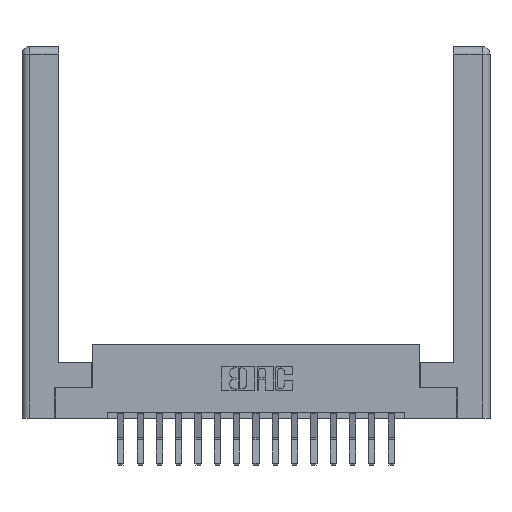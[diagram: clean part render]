
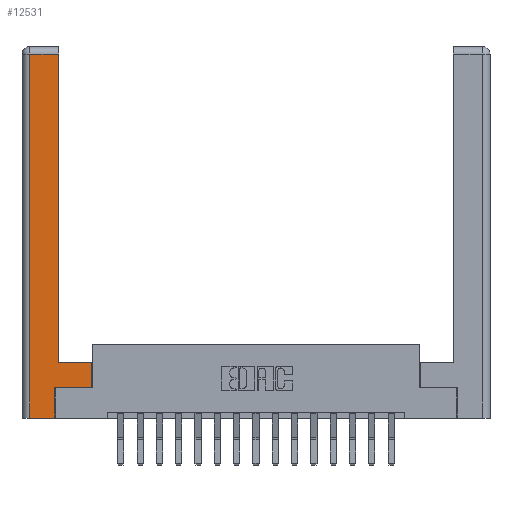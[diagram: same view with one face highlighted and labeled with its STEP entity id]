
A CAD part, top view. The second image highlights one B-rep face of the part: STEP entity #12531.
In plain terms, the highlighted planar face has unit normal (0, 0, 1).
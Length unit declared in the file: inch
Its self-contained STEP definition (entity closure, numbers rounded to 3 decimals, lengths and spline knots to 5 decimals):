
#8 = DIRECTION ( 'NONE',  ( 0., 1., 0. ) ) ;
#208 = ORIENTED_EDGE ( 'NONE', *, *, #5203, .T. ) ;
#360 = DIRECTION ( 'NONE',  ( 0., 1., 0. ) ) ;
#1199 = CARTESIAN_POINT ( 'NONE',  ( 0.295, 3., 0. ) ) ;
#1232 = LINE ( 'NONE', #2982, #1459 ) ;
#1459 = VECTOR ( 'NONE', #15765, 39.37008 ) ;
#1787 = VECTOR ( 'NONE', #8, 39.37008 ) ;
#2088 = VECTOR ( 'NONE', #4106, 39.37008 ) ;
#2419 = VERTEX_POINT ( 'NONE', #6760 ) ;
#2529 = LINE ( 'NONE', #7119, #14407 ) ;
#2982 = CARTESIAN_POINT ( 'NONE',  ( 0.0615, 2.94, 0. ) ) ;
#3118 = DIRECTION ( 'NONE',  ( 1., 0., 0. ) ) ;
#3266 = ORIENTED_EDGE ( 'NONE', *, *, #4541, .T. ) ;
#3797 = VECTOR ( 'NONE', #360, 39.37008 ) ;
#4025 = ORIENTED_EDGE ( 'NONE', *, *, #7799, .T. ) ;
#4106 = DIRECTION ( 'NONE',  ( 1., 0., 0. ) ) ;
#4179 = LINE ( 'NONE', #6961, #13903 ) ;
#4541 = EDGE_CURVE ( 'NONE', #10365, #13304, #2529, .T. ) ;
#4639 = EDGE_CURVE ( 'NONE', #7550, #15956, #9853, .T. ) ;
#4885 = LINE ( 'NONE', #10863, #2088 ) ;
#4930 = EDGE_CURVE ( 'NONE', #5058, #9296, #12443, .T. ) ;
#5058 = VERTEX_POINT ( 'NONE', #12957 ) ;
#5203 = EDGE_CURVE ( 'NONE', #15956, #15890, #11600, .T. ) ;
#5273 = ORIENTED_EDGE ( 'NONE', *, *, #4930, .T. ) ;
#5280 = CARTESIAN_POINT ( 'NONE',  ( 0., 0., 0. ) ) ;
#5290 = EDGE_CURVE ( 'NONE', #13304, #2419, #4885, .T. ) ;
#5510 = CARTESIAN_POINT ( 'NONE',  ( 0.265, 0.245, 0. ) ) ;
#5647 = CARTESIAN_POINT ( 'NONE',  ( 0.265, 0.245, 0. ) ) ;
#6760 = CARTESIAN_POINT ( 'NONE',  ( 0.265, 0., 0. ) ) ;
#6961 = CARTESIAN_POINT ( 'NONE',  ( 0.295, 0.45, 0. ) ) ;
#7119 = CARTESIAN_POINT ( 'NONE',  ( 0.0615, 0., 0. ) ) ;
#7178 = CARTESIAN_POINT ( 'NONE',  ( 0.0615, 0., 0. ) ) ;
#7286 = VECTOR ( 'NONE', #3118, 39.37008 ) ;
#7396 = LINE ( 'NONE', #5510, #1787 ) ;
#7550 = VERTEX_POINT ( 'NONE', #5647 ) ;
#7684 = EDGE_LOOP ( 'NONE', ( #5273, #10714, #3266, #16982, #13764, #8292, #208, #4025 ) ) ;
#7799 = EDGE_CURVE ( 'NONE', #15890, #5058, #4179, .T. ) ;
#7849 = DIRECTION ( 'NONE',  ( 0., 0., -1. ) ) ;
#8134 = EDGE_CURVE ( 'NONE', #2419, #7550, #7396, .T. ) ;
#8217 = DIRECTION ( 'NONE',  ( 0., 1., 0. ) ) ;
#8292 = ORIENTED_EDGE ( 'NONE', *, *, #4639, .T. ) ;
#8752 = VECTOR ( 'NONE', #8217, 39.37008 ) ;
#9296 = VERTEX_POINT ( 'NONE', #9409 ) ;
#9397 = DIRECTION ( 'NONE',  ( -1., 0., 0. ) ) ;
#9409 = CARTESIAN_POINT ( 'NONE',  ( 0.295, 2.94, 0. ) ) ;
#9720 = AXIS2_PLACEMENT_3D ( 'NONE', #5280, #7849, #9397 ) ;
#9769 = DIRECTION ( 'NONE',  ( -1., 0., 0. ) ) ;
#9853 = LINE ( 'NONE', #10058, #7286 ) ;
#10058 = CARTESIAN_POINT ( 'NONE',  ( 0.565, 0.245, 0. ) ) ;
#10365 = VERTEX_POINT ( 'NONE', #17554 ) ;
#10714 = ORIENTED_EDGE ( 'NONE', *, *, #11097, .T. ) ;
#10863 = CARTESIAN_POINT ( 'NONE',  ( 0.265, 0., 0. ) ) ;
#11097 = EDGE_CURVE ( 'NONE', #9296, #10365, #1232, .T. ) ;
#11520 = CARTESIAN_POINT ( 'NONE',  ( 0.565, 0.45, 0. ) ) ;
#11600 = LINE ( 'NONE', #16899, #3797 ) ;
#12443 = LINE ( 'NONE', #1199, #8752 ) ;
#12531 = ADVANCED_FACE ( 'NONE', ( #12674 ), #16316, .F. ) ;
#12674 = FACE_OUTER_BOUND ( 'NONE', #7684, .T. ) ;
#12957 = CARTESIAN_POINT ( 'NONE',  ( 0.295, 0.45, 0. ) ) ;
#13304 = VERTEX_POINT ( 'NONE', #7178 ) ;
#13764 = ORIENTED_EDGE ( 'NONE', *, *, #8134, .T. ) ;
#13765 = DIRECTION ( 'NONE',  ( 0., -1., 0. ) ) ;
#13903 = VECTOR ( 'NONE', #9769, 39.37008 ) ;
#14407 = VECTOR ( 'NONE', #13765, 39.37008 ) ;
#15765 = DIRECTION ( 'NONE',  ( -1., 0., 0. ) ) ;
#15890 = VERTEX_POINT ( 'NONE', #11520 ) ;
#15956 = VERTEX_POINT ( 'NONE', #17368 ) ;
#16316 = PLANE ( 'NONE',  #9720 ) ;
#16899 = CARTESIAN_POINT ( 'NONE',  ( 0.565, 0.45, 0. ) ) ;
#16982 = ORIENTED_EDGE ( 'NONE', *, *, #5290, .T. ) ;
#17368 = CARTESIAN_POINT ( 'NONE',  ( 0.565, 0.245, 0. ) ) ;
#17554 = CARTESIAN_POINT ( 'NONE',  ( 0.0615, 2.94, 0. ) ) ;
